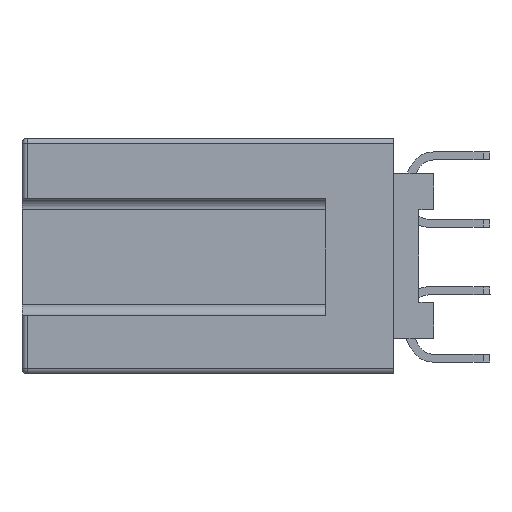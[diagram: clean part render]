
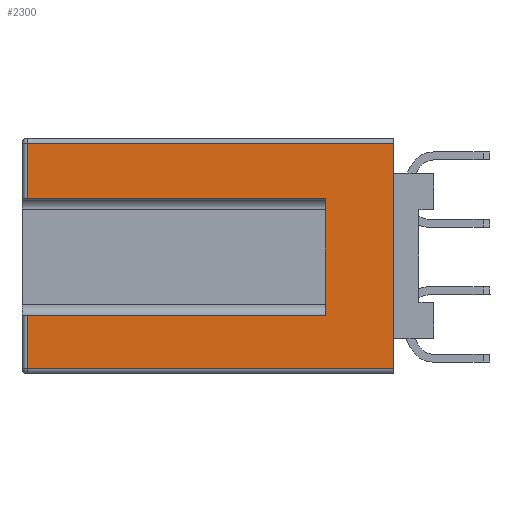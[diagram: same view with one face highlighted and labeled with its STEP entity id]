
A CAD part, left-side view. The second image highlights one B-rep face of the part: STEP entity #2300.
In plain terms, the highlighted planar face has unit normal (-1, 0, 0).
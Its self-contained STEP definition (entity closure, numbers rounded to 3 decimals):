
#221 = LINE ( 'NONE', #3955, #15600 ) ;
#2300 = ADVANCED_FACE ( 'NONE', ( #37938 ), #44921, .F. ) ;
#2846 = VERTEX_POINT ( 'NONE', #5167 ) ;
#3521 = LINE ( 'NONE', #21068, #24768 ) ;
#3955 = CARTESIAN_POINT ( 'NONE',  ( 0., 4.07, -2.28 ) ) ;
#4769 = DIRECTION ( 'NONE',  ( 0., 0., -1. ) ) ;
#5167 = CARTESIAN_POINT ( 'NONE',  ( 0., 4.07, -6.68 ) ) ;
#6382 = VERTEX_POINT ( 'NONE', #37891 ) ;
#7157 = DIRECTION ( 'NONE',  ( 0., 1., 0. ) ) ;
#7882 = EDGE_CURVE ( 'NONE', #19420, #35632, #3521, .T. ) ;
#9803 = CARTESIAN_POINT ( 'NONE',  ( 0., 15.3, -0.2 ) ) ;
#10063 = EDGE_CURVE ( 'NONE', #45443, #41385, #43664, .T. ) ;
#10900 = LINE ( 'NONE', #15278, #43794 ) ;
#11594 = VECTOR ( 'NONE', #26153, 1000. ) ;
#11962 = EDGE_CURVE ( 'NONE', #2846, #6382, #41254, .T. ) ;
#12228 = DIRECTION ( 'NONE',  ( 1., 0., 0. ) ) ;
#15278 = CARTESIAN_POINT ( 'NONE',  ( 0., 15.5, -0.2 ) ) ;
#15600 = VECTOR ( 'NONE', #39951, 1000. ) ;
#15775 = LINE ( 'NONE', #22555, #16125 ) ;
#15784 = CARTESIAN_POINT ( 'NONE',  ( 0., 15.3, -8.68 ) ) ;
#16125 = VECTOR ( 'NONE', #4769, 1000. ) ;
#16163 = LINE ( 'NONE', #41158, #27552 ) ;
#17807 = DIRECTION ( 'NONE',  ( 0., 0., -1. ) ) ;
#18610 = VECTOR ( 'NONE', #23989, 1000. ) ;
#19048 = EDGE_CURVE ( 'NONE', #6382, #38302, #15775, .T. ) ;
#19420 = VERTEX_POINT ( 'NONE', #35388 ) ;
#19717 = ORIENTED_EDGE ( 'NONE', *, *, #7882, .F. ) ;
#21068 = CARTESIAN_POINT ( 'NONE',  ( 0., 1.5, 0. ) ) ;
#21284 = ORIENTED_EDGE ( 'NONE', *, *, #19048, .T. ) ;
#21590 = CARTESIAN_POINT ( 'NONE',  ( 0., 1.5, -8.68 ) ) ;
#22185 = CARTESIAN_POINT ( 'NONE',  ( 0., 15.3, 0. ) ) ;
#22243 = EDGE_CURVE ( 'NONE', #41385, #42859, #221, .T. ) ;
#22555 = CARTESIAN_POINT ( 'NONE',  ( 0., 15.3, 0. ) ) ;
#22806 = ORIENTED_EDGE ( 'NONE', *, *, #27344, .T. ) ;
#23989 = DIRECTION ( 'NONE',  ( 0., 1., 0. ) ) ;
#24768 = VECTOR ( 'NONE', #17807, 1000. ) ;
#26153 = DIRECTION ( 'NONE',  ( 0., 0., -1. ) ) ;
#27344 = EDGE_CURVE ( 'NONE', #38302, #35632, #16163, .T. ) ;
#27552 = VECTOR ( 'NONE', #37211, 1000. ) ;
#27689 = EDGE_CURVE ( 'NONE', #42859, #2846, #44368, .T. ) ;
#27751 = EDGE_LOOP ( 'NONE', ( #21284, #22806, #19717, #45635, #32865, #42923, #32673, #40737 ) ) ;
#30595 = CARTESIAN_POINT ( 'NONE',  ( 0., 4.07, -2.28 ) ) ;
#32673 = ORIENTED_EDGE ( 'NONE', *, *, #27689, .T. ) ;
#32865 = ORIENTED_EDGE ( 'NONE', *, *, #10063, .T. ) ;
#34430 = AXIS2_PLACEMENT_3D ( 'NONE', #44237, #12228, #40734 ) ;
#35388 = CARTESIAN_POINT ( 'NONE',  ( 0., 1.5, -0.2 ) ) ;
#35632 = VERTEX_POINT ( 'NONE', #21590 ) ;
#35769 = VECTOR ( 'NONE', #37384, 1000. ) ;
#36020 = CARTESIAN_POINT ( 'NONE',  ( 0., 15.3, -2.28 ) ) ;
#37211 = DIRECTION ( 'NONE',  ( 0., -1., 0. ) ) ;
#37384 = DIRECTION ( 'NONE',  ( 0., 0., -1. ) ) ;
#37891 = CARTESIAN_POINT ( 'NONE',  ( 0., 15.3, -6.68 ) ) ;
#37938 = FACE_OUTER_BOUND ( 'NONE', #27751, .T. ) ;
#38011 = CARTESIAN_POINT ( 'NONE',  ( 0., 4.07, -6.68 ) ) ;
#38302 = VERTEX_POINT ( 'NONE', #15784 ) ;
#39807 = CARTESIAN_POINT ( 'NONE',  ( 0., 4.07, -2.28 ) ) ;
#39951 = DIRECTION ( 'NONE',  ( 0., -1., 0. ) ) ;
#40734 = DIRECTION ( 'NONE',  ( 0., 0., -1. ) ) ;
#40737 = ORIENTED_EDGE ( 'NONE', *, *, #11962, .T. ) ;
#41158 = CARTESIAN_POINT ( 'NONE',  ( 0., 15.5, -8.68 ) ) ;
#41254 = LINE ( 'NONE', #38011, #18610 ) ;
#41385 = VERTEX_POINT ( 'NONE', #36020 ) ;
#42859 = VERTEX_POINT ( 'NONE', #39807 ) ;
#42923 = ORIENTED_EDGE ( 'NONE', *, *, #22243, .T. ) ;
#43664 = LINE ( 'NONE', #22185, #11594 ) ;
#43794 = VECTOR ( 'NONE', #7157, 1000. ) ;
#44237 = CARTESIAN_POINT ( 'NONE',  ( 0., 15.5, 0. ) ) ;
#44368 = LINE ( 'NONE', #30595, #35769 ) ;
#44921 = PLANE ( 'NONE',  #34430 ) ;
#45443 = VERTEX_POINT ( 'NONE', #9803 ) ;
#45635 = ORIENTED_EDGE ( 'NONE', *, *, #46000, .T. ) ;
#46000 = EDGE_CURVE ( 'NONE', #19420, #45443, #10900, .T. ) ;
